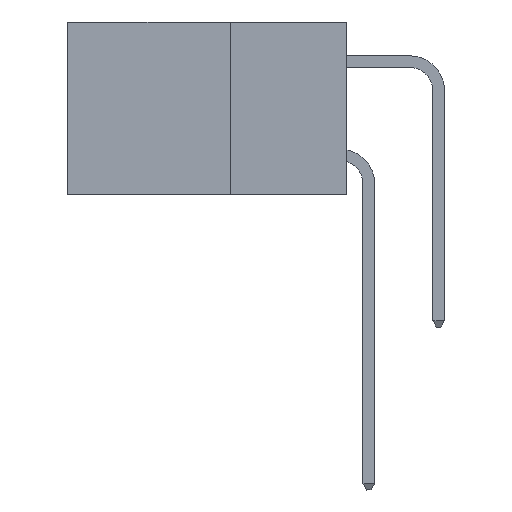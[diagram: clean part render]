
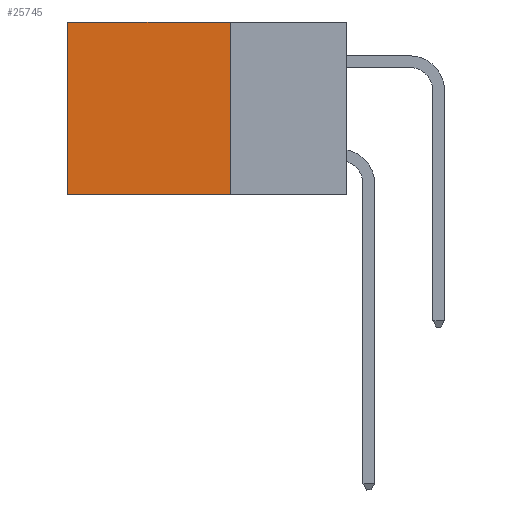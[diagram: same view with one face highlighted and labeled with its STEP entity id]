
A CAD part, left-side view. The second image highlights one B-rep face of the part: STEP entity #25745.
In plain terms, the highlighted planar face has unit normal (-1, 0, 0).
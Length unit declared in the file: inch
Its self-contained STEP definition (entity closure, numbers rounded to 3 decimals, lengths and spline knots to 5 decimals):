
#700 = VECTOR ( 'NONE', #27315, 39.37008 ) ;
#1181 = DIRECTION ( 'NONE',  ( 0., 1., 0. ) ) ;
#1226 = CARTESIAN_POINT ( 'NONE',  ( 0.2875, 0.25, -0.37 ) ) ;
#1817 = VERTEX_POINT ( 'NONE', #1226 ) ;
#1852 = DIRECTION ( 'NONE',  ( 1., 0., 0. ) ) ;
#2369 = CARTESIAN_POINT ( 'NONE',  ( 0.2875, 0.6, 0. ) ) ;
#2467 = DIRECTION ( 'NONE',  ( 0., 0., -1. ) ) ;
#4276 = LINE ( 'NONE', #2369, #28141 ) ;
#4334 = VERTEX_POINT ( 'NONE', #5107 ) ;
#5107 = CARTESIAN_POINT ( 'NONE',  ( 0.2875, 0.6, -0.37 ) ) ;
#6010 = PLANE ( 'NONE',  #11035 ) ;
#6247 = VERTEX_POINT ( 'NONE', #26466 ) ;
#7913 = CARTESIAN_POINT ( 'NONE',  ( 0.2875, 0.25, 0. ) ) ;
#9748 = CARTESIAN_POINT ( 'NONE',  ( 0.2875, 0.25, 0. ) ) ;
#10228 = LINE ( 'NONE', #15666, #27688 ) ;
#10297 = EDGE_CURVE ( 'NONE', #1817, #4334, #18835, .T. ) ;
#10556 = EDGE_LOOP ( 'NONE', ( #18270, #16588, #21045, #12529 ) ) ;
#10939 = DIRECTION ( 'NONE',  ( 0., 0., -1. ) ) ;
#11035 = AXIS2_PLACEMENT_3D ( 'NONE', #24591, #1852, #10939 ) ;
#11044 = FACE_OUTER_BOUND ( 'NONE', #10556, .T. ) ;
#11391 = CARTESIAN_POINT ( 'NONE',  ( 0.2875, 0.25, -0.37 ) ) ;
#12529 = ORIENTED_EDGE ( 'NONE', *, *, #21267, .T. ) ;
#15666 = CARTESIAN_POINT ( 'NONE',  ( 0.2875, 0.25, 0. ) ) ;
#15982 = EDGE_CURVE ( 'NONE', #6247, #4334, #4276, .T. ) ;
#16588 = ORIENTED_EDGE ( 'NONE', *, *, #10297, .F. ) ;
#18270 = ORIENTED_EDGE ( 'NONE', *, *, #15982, .T. ) ;
#18835 = LINE ( 'NONE', #11391, #700 ) ;
#21045 = ORIENTED_EDGE ( 'NONE', *, *, #28226, .F. ) ;
#21267 = EDGE_CURVE ( 'NONE', #26147, #6247, #24356, .T. ) ;
#24356 = LINE ( 'NONE', #7913, #26475 ) ;
#24591 = CARTESIAN_POINT ( 'NONE',  ( 0.2875, 0.25, 0. ) ) ;
#25745 = ADVANCED_FACE ( 'NONE', ( #11044 ), #6010, .F. ) ;
#26147 = VERTEX_POINT ( 'NONE', #9748 ) ;
#26466 = CARTESIAN_POINT ( 'NONE',  ( 0.2875, 0.6, 0. ) ) ;
#26475 = VECTOR ( 'NONE', #1181, 39.37008 ) ;
#27315 = DIRECTION ( 'NONE',  ( 0., 1., 0. ) ) ;
#27688 = VECTOR ( 'NONE', #29072, 39.37008 ) ;
#28141 = VECTOR ( 'NONE', #2467, 39.37008 ) ;
#28226 = EDGE_CURVE ( 'NONE', #26147, #1817, #10228, .T. ) ;
#29072 = DIRECTION ( 'NONE',  ( 0., 0., -1. ) ) ;
